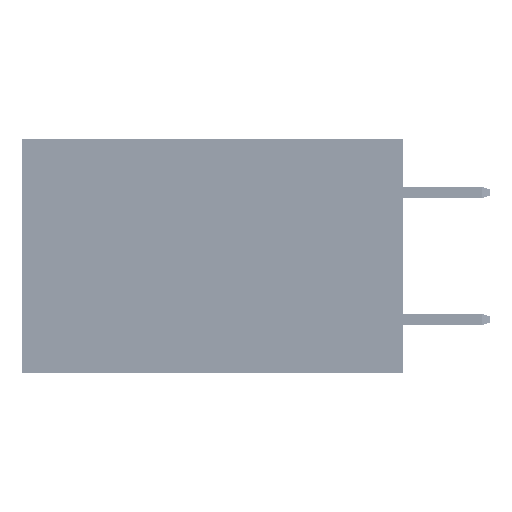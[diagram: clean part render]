
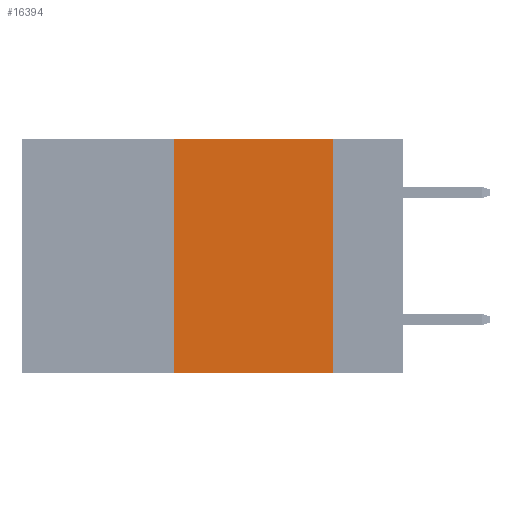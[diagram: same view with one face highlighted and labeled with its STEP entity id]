
A CAD part, left-side view. The second image highlights one B-rep face of the part: STEP entity #16394.
In plain terms, the highlighted planar face has unit normal (-1, 0, 0).
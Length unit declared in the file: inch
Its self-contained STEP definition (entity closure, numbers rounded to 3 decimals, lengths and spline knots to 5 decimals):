
#471 = ORIENTED_EDGE ( 'NONE', *, *, #26423, .F. ) ;
#2205 = CARTESIAN_POINT ( 'NONE',  ( 0., 0.11, 0. ) ) ;
#2724 = DIRECTION ( 'NONE',  ( 0., 0., -1. ) ) ;
#2756 = AXIS2_PLACEMENT_3D ( 'NONE', #20002, #24265, #12494 ) ;
#7707 = CARTESIAN_POINT ( 'NONE',  ( 0., 0.36, 0. ) ) ;
#9983 = CARTESIAN_POINT ( 'NONE',  ( 0., 0.11, 0. ) ) ;
#12494 = DIRECTION ( 'NONE',  ( 0., 0., -1. ) ) ;
#13895 = ORIENTED_EDGE ( 'NONE', *, *, #15063, .F. ) ;
#14432 = CARTESIAN_POINT ( 'NONE',  ( 0., 0.36, 0. ) ) ;
#15063 = EDGE_CURVE ( 'NONE', #36653, #17918, #38157, .T. ) ;
#15129 = CARTESIAN_POINT ( 'NONE',  ( 0., 0.6, 0. ) ) ;
#15278 = LINE ( 'NONE', #35050, #29002 ) ;
#15478 = DIRECTION ( 'NONE',  ( 0., 0., 1. ) ) ;
#16394 = ADVANCED_FACE ( 'NONE', ( #47044 ), #40260, .F. ) ;
#17918 = VERTEX_POINT ( 'NONE', #2205 ) ;
#20002 = CARTESIAN_POINT ( 'NONE',  ( 0., 0.6, 0. ) ) ;
#21300 = VECTOR ( 'NONE', #2724, 39.37008 ) ;
#22673 = VECTOR ( 'NONE', #41788, 39.37008 ) ;
#23798 = DIRECTION ( 'NONE',  ( 0., -1., 0. ) ) ;
#24265 = DIRECTION ( 'NONE',  ( 1., 0., 0. ) ) ;
#24470 = EDGE_LOOP ( 'NONE', ( #35877, #13895, #471, #30725 ) ) ;
#26054 = VERTEX_POINT ( 'NONE', #46088 ) ;
#26423 = EDGE_CURVE ( 'NONE', #26054, #36653, #29993, .T. ) ;
#29002 = VECTOR ( 'NONE', #23798, 39.37008 ) ;
#29993 = LINE ( 'NONE', #7707, #45858 ) ;
#30725 = ORIENTED_EDGE ( 'NONE', *, *, #38328, .T. ) ;
#35050 = CARTESIAN_POINT ( 'NONE',  ( 0., 0.6, -0.37 ) ) ;
#35877 = ORIENTED_EDGE ( 'NONE', *, *, #44562, .F. ) ;
#36653 = VERTEX_POINT ( 'NONE', #14432 ) ;
#37000 = LINE ( 'NONE', #9983, #21300 ) ;
#38157 = LINE ( 'NONE', #15129, #22673 ) ;
#38328 = EDGE_CURVE ( 'NONE', #26054, #44825, #15278, .T. ) ;
#40260 = PLANE ( 'NONE',  #2756 ) ;
#41788 = DIRECTION ( 'NONE',  ( 0., -1., 0. ) ) ;
#44562 = EDGE_CURVE ( 'NONE', #17918, #44825, #37000, .T. ) ;
#44825 = VERTEX_POINT ( 'NONE', #46995 ) ;
#45858 = VECTOR ( 'NONE', #15478, 39.37008 ) ;
#46088 = CARTESIAN_POINT ( 'NONE',  ( 0., 0.36, -0.37 ) ) ;
#46995 = CARTESIAN_POINT ( 'NONE',  ( 0., 0.11, -0.37 ) ) ;
#47044 = FACE_OUTER_BOUND ( 'NONE', #24470, .T. ) ;
